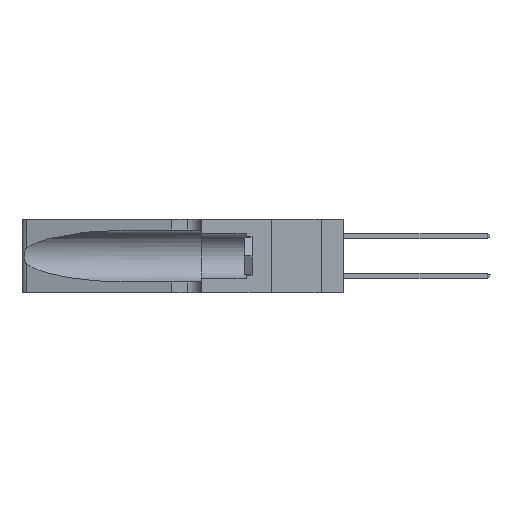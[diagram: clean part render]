
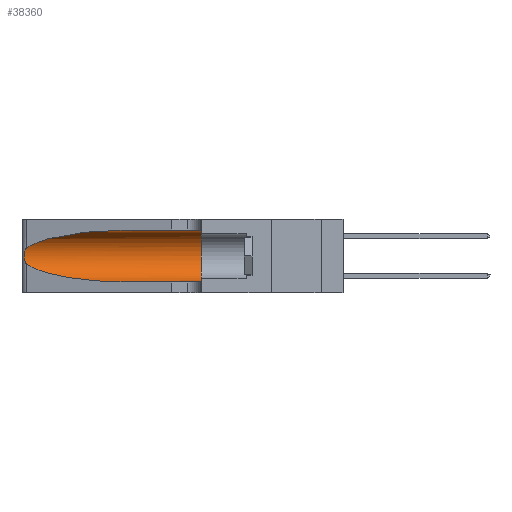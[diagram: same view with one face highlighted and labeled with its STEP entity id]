
A CAD part, left-side view. The second image highlights one B-rep face of the part: STEP entity #38360.
In plain terms, the highlighted cylindrical face has radius 3.308 mm (diameter 6.617 mm), a partial arc.
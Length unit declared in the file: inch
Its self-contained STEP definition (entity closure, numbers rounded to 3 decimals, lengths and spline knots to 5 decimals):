
#529 = B_SPLINE_CURVE_WITH_KNOTS ( 'NONE', 3,
 ( #26183, #29185, #8403, #32202, #14408, #35184, #17358, #38183, #20318, #2566, #23308, #5547, #26318, #8537 ),
 .UNSPECIFIED., .F., .F.,
 ( 4, 2, 2, 2, 2, 2, 4 ),
 ( 0., 0.00027, 0.00053, 0.00107, 0.0016, 0.00187, 0.00214 ),
 .UNSPECIFIED. ) ;
#530 = VERTEX_POINT ( 'NONE', #32152 ) ;
#836 = DIRECTION ( 'NONE',  ( 0., 0., 1. ) ) ;
#1734 = FACE_OUTER_BOUND ( 'NONE', #2572, .T. ) ;
#2566 = CARTESIAN_POINT ( 'NONE',  ( 0.25856, 1.23593, 0.16098 ) ) ;
#2572 = EDGE_LOOP ( 'NONE', ( #6617, #33020, #35127, #13151, #6289, #30232 ) ) ;
#2613 = VERTEX_POINT ( 'NONE', #23440 ) ;
#3432 =( BOUNDED_CURVE ( )  B_SPLINE_CURVE ( 3, ( #32517, #14721, #35503, #17680 ),
 .UNSPECIFIED., .F., .T. ) 
 B_SPLINE_CURVE_WITH_KNOTS ( ( 4, 4 ),
 ( 1.5708, 2.84003 ),
 .UNSPECIFIED. ) 
 CURVE ( )  GEOMETRIC_REPRESENTATION_ITEM ( )  RATIONAL_B_SPLINE_CURVE ( ( 1., 0.87, 0.87, 1. ) ) 
 REPRESENTATION_ITEM ( '' )  );
#5547 = CARTESIAN_POINT ( 'NONE',  ( 0.25639, 1.23186, 0.15144 ) ) ;
#6289 = ORIENTED_EDGE ( 'NONE', *, *, #35224, .F. ) ;
#6617 = ORIENTED_EDGE ( 'NONE', *, *, #22712, .T. ) ;
#7380 = CARTESIAN_POINT ( 'NONE',  ( 0.1305, 1.61858, 0.05475 ) ) ;
#7454 = DIRECTION ( 'NONE',  ( 0., -1., 0. ) ) ;
#7568 = EDGE_CURVE ( 'NONE', #7582, #29476, #529, .T. ) ;
#7582 = VERTEX_POINT ( 'NONE', #38306 ) ;
#8403 = CARTESIAN_POINT ( 'NONE',  ( 0.25639, 1.23184, 0.21858 ) ) ;
#8537 = CARTESIAN_POINT ( 'NONE',  ( 0.25487, 1.22718, 0.14631 ) ) ;
#11910 = DIRECTION ( 'NONE',  ( 0., -1., 0. ) ) ;
#12632 = AXIS2_PLACEMENT_3D ( 'NONE', #36474, #18651, #836 ) ;
#13151 = ORIENTED_EDGE ( 'NONE', *, *, #29566, .T. ) ;
#13958 = AXIS2_PLACEMENT_3D ( 'NONE', #34240, #7454, #16412 ) ;
#14176 = EDGE_CURVE ( 'NONE', #29476, #22966, #21244, .T. ) ;
#14408 = CARTESIAN_POINT ( 'NONE',  ( 0.25854, 1.2359, 0.20912 ) ) ;
#14721 = CARTESIAN_POINT ( 'NONE',  ( 0.18966, 0.96281, 0.31525 ) ) ;
#14873 = CARTESIAN_POINT ( 'NONE',  ( 0.1305, 0.72297, 0.05475 ) ) ;
#16412 = DIRECTION ( 'NONE',  ( 0., 0., -1. ) ) ;
#17358 = CARTESIAN_POINT ( 'NONE',  ( 0.26075, 1.23896, 0.19203 ) ) ;
#17680 = CARTESIAN_POINT ( 'NONE',  ( 0.25487, 1.22718, 0.22369 ) ) ;
#18651 = DIRECTION ( 'NONE',  ( 0., 1., 0. ) ) ;
#19223 = LINE ( 'NONE', #23692, #33219 ) ;
#20318 = CARTESIAN_POINT ( 'NONE',  ( 0.26017, 1.23833, 0.17102 ) ) ;
#21244 =( BOUNDED_CURVE ( )  B_SPLINE_CURVE ( 3, ( #29684, #26668, #32675, #14873 ),
 .UNSPECIFIED., .F., .F. ) 
 B_SPLINE_CURVE_WITH_KNOTS ( ( 4, 4 ),
 ( 3.44316, 4.71239 ),
 .UNSPECIFIED. ) 
 CURVE ( )  GEOMETRIC_REPRESENTATION_ITEM ( )  RATIONAL_B_SPLINE_CURVE ( ( 1., 0.87, 0.87, 1. ) ) 
 REPRESENTATION_ITEM ( '' )  );
#22712 = EDGE_CURVE ( 'NONE', #2613, #7582, #3432, .T. ) ;
#22966 = VERTEX_POINT ( 'NONE', #30666 ) ;
#23308 = CARTESIAN_POINT ( 'NONE',  ( 0.25789, 1.23486, 0.15765 ) ) ;
#23440 = CARTESIAN_POINT ( 'NONE',  ( 0.1305, 0.72297, 0.31525 ) ) ;
#23692 = CARTESIAN_POINT ( 'NONE',  ( 0.1305, 1.61858, 0.31525 ) ) ;
#24207 = VECTOR ( 'NONE', #25195, 39.37008 ) ;
#24510 = CYLINDRICAL_SURFACE ( 'NONE', #13958, 0.13025 ) ;
#25195 = DIRECTION ( 'NONE',  ( 0., -1., 0. ) ) ;
#26183 = CARTESIAN_POINT ( 'NONE',  ( 0.25487, 1.22718, 0.22369 ) ) ;
#26318 = CARTESIAN_POINT ( 'NONE',  ( 0.25555, 1.22993, 0.14849 ) ) ;
#26668 = CARTESIAN_POINT ( 'NONE',  ( 0.2373, 1.15595, 0.08982 ) ) ;
#29185 = CARTESIAN_POINT ( 'NONE',  ( 0.25555, 1.22994, 0.2215 ) ) ;
#29476 = VERTEX_POINT ( 'NONE', #30812 ) ;
#29566 = EDGE_CURVE ( 'NONE', #22966, #30251, #33063, .T. ) ;
#29684 = CARTESIAN_POINT ( 'NONE',  ( 0.25487, 1.22718, 0.14631 ) ) ;
#30232 = ORIENTED_EDGE ( 'NONE', *, *, #37591, .F. ) ;
#30251 = VERTEX_POINT ( 'NONE', #37789 ) ;
#30666 = CARTESIAN_POINT ( 'NONE',  ( 0.1305, 0.72297, 0.05475 ) ) ;
#30812 = CARTESIAN_POINT ( 'NONE',  ( 0.25487, 1.22718, 0.14631 ) ) ;
#32152 = CARTESIAN_POINT ( 'NONE',  ( 0.1305, 0.35, 0.31525 ) ) ;
#32202 = CARTESIAN_POINT ( 'NONE',  ( 0.25787, 1.23484, 0.2124 ) ) ;
#32517 = CARTESIAN_POINT ( 'NONE',  ( 0.1305, 0.72297, 0.31525 ) ) ;
#32675 = CARTESIAN_POINT ( 'NONE',  ( 0.18966, 0.96281, 0.05475 ) ) ;
#33020 = ORIENTED_EDGE ( 'NONE', *, *, #7568, .T. ) ;
#33063 = LINE ( 'NONE', #7380, #24207 ) ;
#33219 = VECTOR ( 'NONE', #11910, 39.37008 ) ;
#34240 = CARTESIAN_POINT ( 'NONE',  ( 0.1305, 1.61858, 0.185 ) ) ;
#34348 = CIRCLE ( 'NONE', #12632, 0.13025 ) ;
#35127 = ORIENTED_EDGE ( 'NONE', *, *, #14176, .T. ) ;
#35184 = CARTESIAN_POINT ( 'NONE',  ( 0.26018, 1.23835, 0.19895 ) ) ;
#35224 = EDGE_CURVE ( 'NONE', #530, #30251, #34348, .T. ) ;
#35503 = CARTESIAN_POINT ( 'NONE',  ( 0.2373, 1.15595, 0.28018 ) ) ;
#36474 = CARTESIAN_POINT ( 'NONE',  ( 0.1305, 0.35, 0.185 ) ) ;
#37591 = EDGE_CURVE ( 'NONE', #2613, #530, #19223, .T. ) ;
#37789 = CARTESIAN_POINT ( 'NONE',  ( 0.1305, 0.35, 0.05475 ) ) ;
#38183 = CARTESIAN_POINT ( 'NONE',  ( 0.26075, 1.23896, 0.178 ) ) ;
#38306 = CARTESIAN_POINT ( 'NONE',  ( 0.25487, 1.22718, 0.22369 ) ) ;
#38360 = ADVANCED_FACE ( 'NONE', ( #1734 ), #24510, .F. ) ;
